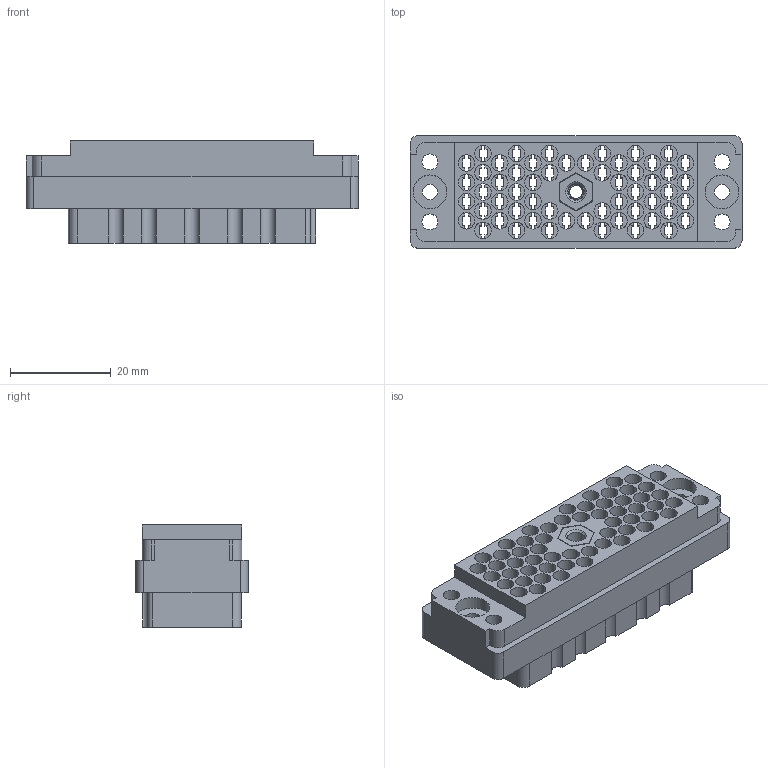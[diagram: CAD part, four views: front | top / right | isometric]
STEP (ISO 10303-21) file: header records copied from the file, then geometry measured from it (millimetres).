
FILE_DESCRIPTION (( 'STEP AP203' ), '1' );
FILE_NAME ('516-056-000-406.STEP', '2020-03-05T19:55:49', ( '' ), ( '' ), 'SwSTEP 2.0', 'SolidWorks 2016', '' );
FILE_SCHEMA (( 'CONFIG_CONTROL_DESIGN' ));
Length unit declared in the file: inch
Products named in the file (3): 516 Part Receptacle_056; 516-252-035-100_516-252-035-100; 516-056-000-406
Assembly tree (2 placements, depth 2):
  516-056-000-406
    516 Part Receptacle_056
    516-252-035-100_516-252-035-100
Bounding box: 65.84 x 22.25 x 20.27 mm (x, y, z)
Volume: 14129.7 mm3; surface area: 20130.5 mm2
Topology: 2 solids, 2 shells, 1319 faces, 3878 edges, 2582 vertices
Faces by surface type: plane 904, cylinder 397, cone 12, bspline 6
Entity records: 46777 total; most frequent: CARTESIAN_POINT 10230, ORIENTED_EDGE 7756, DIRECTION 7470, EDGE_CURVE 3878, LINE 2822, VECTOR 2822, VERTEX_POINT 2582, AXIS2_PLACEMENT_3D 2324
